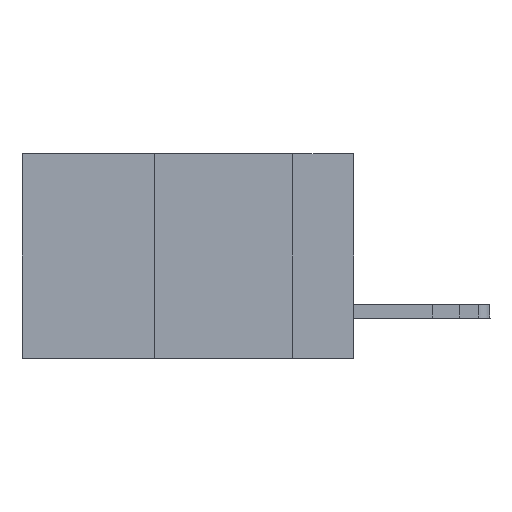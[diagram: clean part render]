
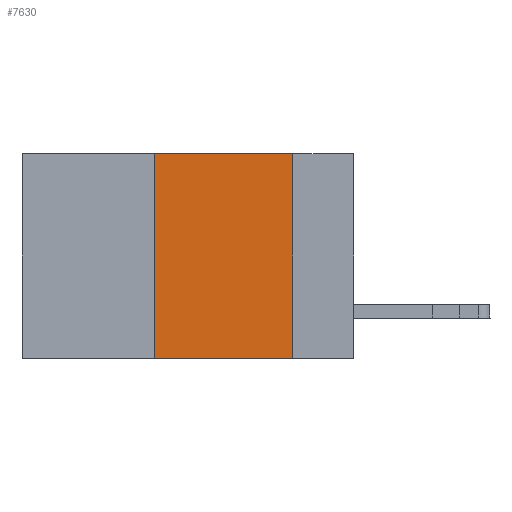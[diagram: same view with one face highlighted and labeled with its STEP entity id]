
A CAD part, left-side view. The second image highlights one B-rep face of the part: STEP entity #7630.
In plain terms, the highlighted planar face has unit normal (-1, 0, 0).
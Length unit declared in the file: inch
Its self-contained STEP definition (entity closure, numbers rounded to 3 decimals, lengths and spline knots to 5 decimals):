
#715 = CARTESIAN_POINT ( 'NONE',  ( 0., 0.11, 0. ) ) ;
#946 = EDGE_LOOP ( 'NONE', ( #2127, #9130, #6387, #14133 ) ) ;
#1482 = DIRECTION ( 'NONE',  ( 0., 0., -1. ) ) ;
#1818 = CARTESIAN_POINT ( 'NONE',  ( 0., 0.11, 0. ) ) ;
#2127 = ORIENTED_EDGE ( 'NONE', *, *, #9040, .F. ) ;
#2150 = CARTESIAN_POINT ( 'NONE',  ( 0., 0.11, -0.37 ) ) ;
#2159 = VERTEX_POINT ( 'NONE', #2150 ) ;
#2540 = EDGE_CURVE ( 'NONE', #14235, #12435, #6816, .T. ) ;
#2656 = FACE_OUTER_BOUND ( 'NONE', #946, .T. ) ;
#2876 = VECTOR ( 'NONE', #10449, 39.37008 ) ;
#3215 = DIRECTION ( 'NONE',  ( 0., 0., -1. ) ) ;
#4235 = CARTESIAN_POINT ( 'NONE',  ( 0., 0.6, 0. ) ) ;
#4393 = VERTEX_POINT ( 'NONE', #5441 ) ;
#5006 = EDGE_CURVE ( 'NONE', #4393, #14235, #7922, .T. ) ;
#5441 = CARTESIAN_POINT ( 'NONE',  ( 0., 0.36, -0.37 ) ) ;
#5463 = CARTESIAN_POINT ( 'NONE',  ( 0., 0.6, -0.37 ) ) ;
#5701 = LINE ( 'NONE', #5463, #2876 ) ;
#6387 = ORIENTED_EDGE ( 'NONE', *, *, #5006, .F. ) ;
#6749 = DIRECTION ( 'NONE',  ( 0., 0., 1. ) ) ;
#6816 = LINE ( 'NONE', #4235, #8076 ) ;
#7417 = PLANE ( 'NONE',  #13191 ) ;
#7630 = ADVANCED_FACE ( 'NONE', ( #2656 ), #7417, .F. ) ;
#7922 = LINE ( 'NONE', #12664, #13159 ) ;
#8076 = VECTOR ( 'NONE', #8992, 39.37008 ) ;
#8992 = DIRECTION ( 'NONE',  ( 0., -1., 0. ) ) ;
#9040 = EDGE_CURVE ( 'NONE', #12435, #2159, #10236, .T. ) ;
#9130 = ORIENTED_EDGE ( 'NONE', *, *, #2540, .F. ) ;
#9747 = CARTESIAN_POINT ( 'NONE',  ( 0., 0.6, 0. ) ) ;
#10236 = LINE ( 'NONE', #715, #11939 ) ;
#10449 = DIRECTION ( 'NONE',  ( 0., -1., 0. ) ) ;
#10682 = EDGE_CURVE ( 'NONE', #4393, #2159, #5701, .T. ) ;
#11939 = VECTOR ( 'NONE', #3215, 39.37008 ) ;
#12435 = VERTEX_POINT ( 'NONE', #1818 ) ;
#12664 = CARTESIAN_POINT ( 'NONE',  ( 0., 0.36, 0. ) ) ;
#12960 = CARTESIAN_POINT ( 'NONE',  ( 0., 0.36, 0. ) ) ;
#13159 = VECTOR ( 'NONE', #6749, 39.37008 ) ;
#13191 = AXIS2_PLACEMENT_3D ( 'NONE', #9747, #14740, #1482 ) ;
#14133 = ORIENTED_EDGE ( 'NONE', *, *, #10682, .T. ) ;
#14235 = VERTEX_POINT ( 'NONE', #12960 ) ;
#14740 = DIRECTION ( 'NONE',  ( 1., 0., 0. ) ) ;
